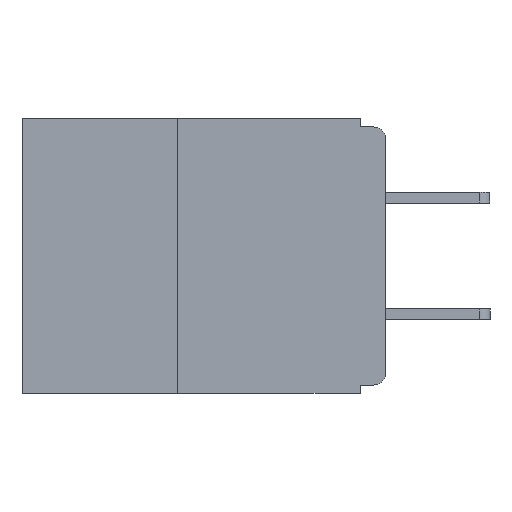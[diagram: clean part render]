
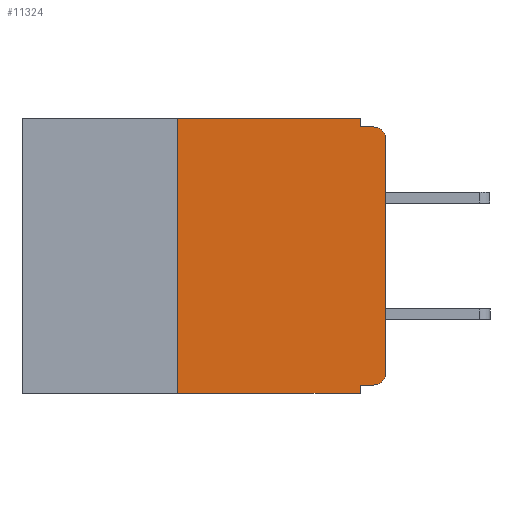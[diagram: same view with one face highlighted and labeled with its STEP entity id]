
A CAD part, left-side view. The second image highlights one B-rep face of the part: STEP entity #11324.
In plain terms, the highlighted planar face has unit normal (-1, 0, 0).
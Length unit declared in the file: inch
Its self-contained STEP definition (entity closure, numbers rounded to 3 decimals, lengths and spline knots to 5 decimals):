
#578 = ORIENTED_EDGE ( 'NONE', *, *, #20579, .F. ) ;
#888 = VECTOR ( 'NONE', #6238, 39.37008 ) ;
#1218 = ORIENTED_EDGE ( 'NONE', *, *, #23047, .F. ) ;
#1735 = DIRECTION ( 'NONE',  ( 0., 0., 1. ) ) ;
#1864 = CARTESIAN_POINT ( 'NONE',  ( 0., 0., 0. ) ) ;
#2212 = DIRECTION ( 'NONE',  ( -1., 0., 0. ) ) ;
#2644 = EDGE_CURVE ( 'NONE', #8394, #5444, #18586, .T. ) ;
#3436 = VERTEX_POINT ( 'NONE', #19888 ) ;
#3460 = CIRCLE ( 'NONE', #6106, 0.015 ) ;
#3571 = LINE ( 'NONE', #12221, #20033 ) ;
#3603 = CARTESIAN_POINT ( 'NONE',  ( 0., 0.015, -0.01 ) ) ;
#3631 = VECTOR ( 'NONE', #17885, 39.37008 ) ;
#4238 = CARTESIAN_POINT ( 'NONE',  ( 0., 0.031, -0.33 ) ) ;
#4419 = VECTOR ( 'NONE', #19402, 39.37008 ) ;
#4759 = ORIENTED_EDGE ( 'NONE', *, *, #16710, .F. ) ;
#5444 = VERTEX_POINT ( 'NONE', #3603 ) ;
#6015 = ORIENTED_EDGE ( 'NONE', *, *, #13421, .F. ) ;
#6106 = AXIS2_PLACEMENT_3D ( 'NONE', #20797, #9069, #22649 ) ;
#6238 = DIRECTION ( 'NONE',  ( 0., 0., -1. ) ) ;
#6686 = CARTESIAN_POINT ( 'NONE',  ( 0., 0.031, -0.32 ) ) ;
#6692 = CARTESIAN_POINT ( 'NONE',  ( 0., 0.437, 0. ) ) ;
#6758 = CARTESIAN_POINT ( 'NONE',  ( 0., 0.015, -0.32 ) ) ;
#6840 = LINE ( 'NONE', #19229, #12149 ) ;
#7196 = FACE_OUTER_BOUND ( 'NONE', #10735, .T. ) ;
#8073 = EDGE_CURVE ( 'NONE', #9009, #15075, #3571, .T. ) ;
#8394 = VERTEX_POINT ( 'NONE', #15147 ) ;
#8794 = VERTEX_POINT ( 'NONE', #21823 ) ;
#9009 = VERTEX_POINT ( 'NONE', #6758 ) ;
#9069 = DIRECTION ( 'NONE',  ( -1., 0., 0. ) ) ;
#9736 = CARTESIAN_POINT ( 'NONE',  ( 0., 0.015, -0.025 ) ) ;
#10092 = ORIENTED_EDGE ( 'NONE', *, *, #25326, .F. ) ;
#10172 = VECTOR ( 'NONE', #1735, 39.37008 ) ;
#10715 = DIRECTION ( 'NONE',  ( 0., 0., -1. ) ) ;
#10735 = EDGE_LOOP ( 'NONE', ( #11974, #12599, #6015, #1218, #10092, #578, #14782, #4759, #14141, #19332 ) ) ;
#11324 = ADVANCED_FACE ( 'NONE', ( #7196 ), #12639, .F. ) ;
#11360 = LINE ( 'NONE', #16908, #21091 ) ;
#11396 = VERTEX_POINT ( 'NONE', #22390 ) ;
#11974 = ORIENTED_EDGE ( 'NONE', *, *, #19967, .T. ) ;
#12149 = VECTOR ( 'NONE', #24778, 39.37008 ) ;
#12221 = CARTESIAN_POINT ( 'NONE',  ( 0., 0., -0.32 ) ) ;
#12599 = ORIENTED_EDGE ( 'NONE', *, *, #2644, .T. ) ;
#12639 = PLANE ( 'NONE',  #21369 ) ;
#13421 = EDGE_CURVE ( 'NONE', #8794, #5444, #6840, .T. ) ;
#13931 = CARTESIAN_POINT ( 'NONE',  ( 0., 0.25, -0.33 ) ) ;
#14141 = ORIENTED_EDGE ( 'NONE', *, *, #8073, .F. ) ;
#14662 = AXIS2_PLACEMENT_3D ( 'NONE', #9736, #2212, #25189 ) ;
#14782 = ORIENTED_EDGE ( 'NONE', *, *, #19313, .T. ) ;
#15075 = VERTEX_POINT ( 'NONE', #6686 ) ;
#15147 = CARTESIAN_POINT ( 'NONE',  ( 0., 0., -0.025 ) ) ;
#15907 = CARTESIAN_POINT ( 'NONE',  ( 0., 0.437, -0.33 ) ) ;
#16060 = LINE ( 'NONE', #25130, #10172 ) ;
#16710 = EDGE_CURVE ( 'NONE', #15075, #19565, #16914, .T. ) ;
#16908 = CARTESIAN_POINT ( 'NONE',  ( 0., 0.437, 0. ) ) ;
#16914 = LINE ( 'NONE', #4238, #888 ) ;
#17448 = CARTESIAN_POINT ( 'NONE',  ( 0., 0.031, 0. ) ) ;
#17868 = DIRECTION ( 'NONE',  ( 0., 0., 1. ) ) ;
#17885 = DIRECTION ( 'NONE',  ( 0., -1., 0. ) ) ;
#18169 = CARTESIAN_POINT ( 'NONE',  ( 0., 0.25, 0. ) ) ;
#18586 = CIRCLE ( 'NONE', #14662, 0.015 ) ;
#18855 = DIRECTION ( 'NONE',  ( 0., -1., 0. ) ) ;
#19149 = LINE ( 'NONE', #1864, #23515 ) ;
#19229 = CARTESIAN_POINT ( 'NONE',  ( 0., 0., -0.01 ) ) ;
#19313 = EDGE_CURVE ( 'NONE', #23173, #19565, #19491, .T. ) ;
#19332 = ORIENTED_EDGE ( 'NONE', *, *, #22900, .T. ) ;
#19402 = DIRECTION ( 'NONE',  ( 0., 0., -1. ) ) ;
#19491 = LINE ( 'NONE', #15907, #3631 ) ;
#19565 = VERTEX_POINT ( 'NONE', #22375 ) ;
#19888 = CARTESIAN_POINT ( 'NONE',  ( 0., 0., -0.305 ) ) ;
#19967 = EDGE_CURVE ( 'NONE', #3436, #8394, #19149, .T. ) ;
#20033 = VECTOR ( 'NONE', #23704, 39.37008 ) ;
#20211 = LINE ( 'NONE', #17448, #4419 ) ;
#20579 = EDGE_CURVE ( 'NONE', #23173, #20758, #16060, .T. ) ;
#20758 = VERTEX_POINT ( 'NONE', #18169 ) ;
#20797 = CARTESIAN_POINT ( 'NONE',  ( 0., 0.015, -0.305 ) ) ;
#21091 = VECTOR ( 'NONE', #18855, 39.37008 ) ;
#21369 = AXIS2_PLACEMENT_3D ( 'NONE', #6692, #22307, #10715 ) ;
#21823 = CARTESIAN_POINT ( 'NONE',  ( 0., 0.031, -0.01 ) ) ;
#22307 = DIRECTION ( 'NONE',  ( 1., 0., 0. ) ) ;
#22375 = CARTESIAN_POINT ( 'NONE',  ( 0., 0.031, -0.33 ) ) ;
#22390 = CARTESIAN_POINT ( 'NONE',  ( 0., 0.031, 0. ) ) ;
#22649 = DIRECTION ( 'NONE',  ( 0., 0., -1. ) ) ;
#22900 = EDGE_CURVE ( 'NONE', #9009, #3436, #3460, .T. ) ;
#23047 = EDGE_CURVE ( 'NONE', #11396, #8794, #20211, .T. ) ;
#23173 = VERTEX_POINT ( 'NONE', #13931 ) ;
#23515 = VECTOR ( 'NONE', #17868, 39.37008 ) ;
#23704 = DIRECTION ( 'NONE',  ( 0., 1., 0. ) ) ;
#24778 = DIRECTION ( 'NONE',  ( 0., -1., 0. ) ) ;
#25130 = CARTESIAN_POINT ( 'NONE',  ( 0., 0.25, -0.33 ) ) ;
#25189 = DIRECTION ( 'NONE',  ( 0., 0., -1. ) ) ;
#25326 = EDGE_CURVE ( 'NONE', #20758, #11396, #11360, .T. ) ;
